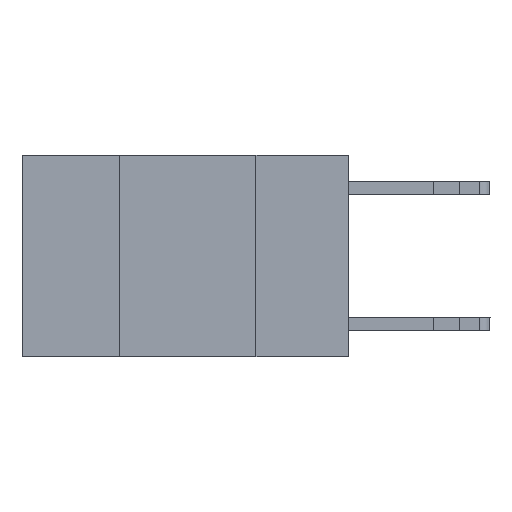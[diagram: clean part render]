
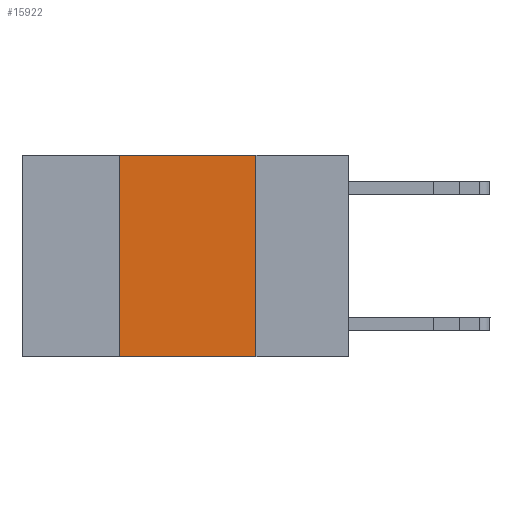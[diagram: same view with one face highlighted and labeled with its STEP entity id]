
A CAD part, left-side view. The second image highlights one B-rep face of the part: STEP entity #15922.
In plain terms, the highlighted planar face has unit normal (-1, 0, 0).
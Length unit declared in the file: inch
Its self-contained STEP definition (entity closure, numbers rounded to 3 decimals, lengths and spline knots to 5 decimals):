
#571 = CARTESIAN_POINT ( 'NONE',  ( 0., 0.42, 0. ) ) ;
#1540 = CARTESIAN_POINT ( 'NONE',  ( 0., 0.6, -0.37 ) ) ;
#3084 = VECTOR ( 'NONE', #23197, 39.37008 ) ;
#3569 = LINE ( 'NONE', #571, #3084 ) ;
#3736 = DIRECTION ( 'NONE',  ( 0., -1., 0. ) ) ;
#3833 = CARTESIAN_POINT ( 'NONE',  ( 0., 0.6, 0. ) ) ;
#3930 = PLANE ( 'NONE',  #9058 ) ;
#4023 = CARTESIAN_POINT ( 'NONE',  ( 0., 0.42, -0.37 ) ) ;
#6104 = DIRECTION ( 'NONE',  ( 0., 0., -1. ) ) ;
#7393 = DIRECTION ( 'NONE',  ( 0., 0., -1. ) ) ;
#7640 = VECTOR ( 'NONE', #7834, 39.37008 ) ;
#7717 = LINE ( 'NONE', #25901, #7640 ) ;
#7834 = DIRECTION ( 'NONE',  ( 0., -1., 0. ) ) ;
#8070 = VECTOR ( 'NONE', #7393, 39.37008 ) ;
#8400 = CARTESIAN_POINT ( 'NONE',  ( 0., 0.17, -0.37 ) ) ;
#8834 = LINE ( 'NONE', #25488, #8070 ) ;
#9058 = AXIS2_PLACEMENT_3D ( 'NONE', #3833, #18381, #6104 ) ;
#9192 = VERTEX_POINT ( 'NONE', #4023 ) ;
#11545 = CARTESIAN_POINT ( 'NONE',  ( 0., 0.17, 0. ) ) ;
#11956 = VERTEX_POINT ( 'NONE', #11545 ) ;
#12685 = FACE_OUTER_BOUND ( 'NONE', #12917, .T. ) ;
#12769 = EDGE_CURVE ( 'NONE', #9192, #19163, #15566, .T. ) ;
#12917 = EDGE_LOOP ( 'NONE', ( #24542, #24652, #24933, #25178 ) ) ;
#15542 = VECTOR ( 'NONE', #3736, 39.37008 ) ;
#15566 = LINE ( 'NONE', #1540, #15542 ) ;
#15922 = ADVANCED_FACE ( 'NONE', ( #12685 ), #3930, .F. ) ;
#16518 = EDGE_CURVE ( 'NONE', #25666, #11956, #7717, .T. ) ;
#18172 = EDGE_CURVE ( 'NONE', #9192, #25666, #3569, .T. ) ;
#18252 = CARTESIAN_POINT ( 'NONE',  ( 0., 0.42, 0. ) ) ;
#18381 = DIRECTION ( 'NONE',  ( 1., 0., 0. ) ) ;
#19163 = VERTEX_POINT ( 'NONE', #8400 ) ;
#19542 = EDGE_CURVE ( 'NONE', #11956, #19163, #8834, .T. ) ;
#23197 = DIRECTION ( 'NONE',  ( 0., 0., 1. ) ) ;
#24542 = ORIENTED_EDGE ( 'NONE', *, *, #19542, .F. ) ;
#24652 = ORIENTED_EDGE ( 'NONE', *, *, #16518, .F. ) ;
#24933 = ORIENTED_EDGE ( 'NONE', *, *, #18172, .F. ) ;
#25178 = ORIENTED_EDGE ( 'NONE', *, *, #12769, .T. ) ;
#25488 = CARTESIAN_POINT ( 'NONE',  ( 0., 0.17, 0. ) ) ;
#25666 = VERTEX_POINT ( 'NONE', #18252 ) ;
#25901 = CARTESIAN_POINT ( 'NONE',  ( 0., 0.6, 0. ) ) ;
